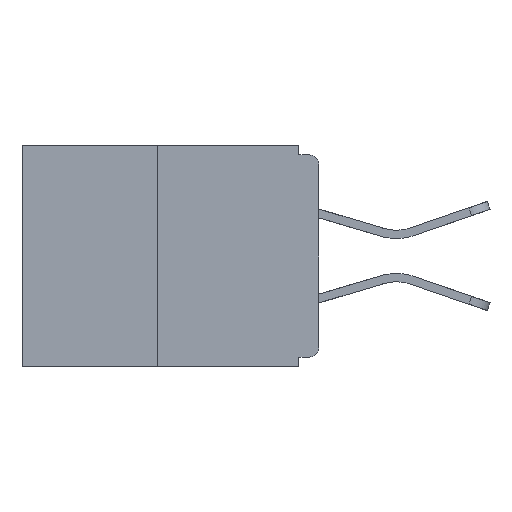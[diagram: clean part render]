
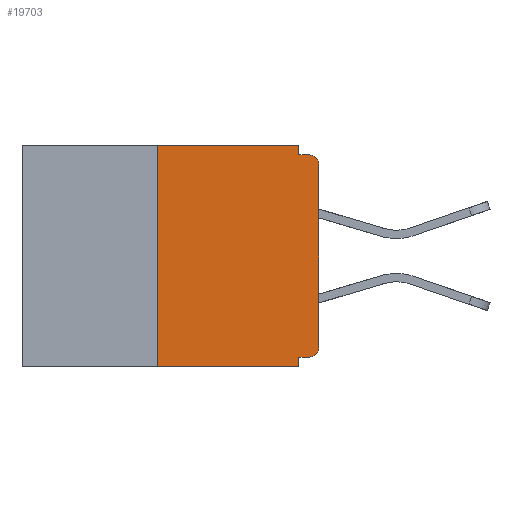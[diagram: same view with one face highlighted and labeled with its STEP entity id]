
A CAD part, left-side view. The second image highlights one B-rep face of the part: STEP entity #19703.
In plain terms, the highlighted planar face has unit normal (-1, 0, 0).
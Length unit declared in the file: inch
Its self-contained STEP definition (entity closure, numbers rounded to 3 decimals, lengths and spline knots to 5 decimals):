
#94 = EDGE_CURVE ( 'NONE', #18329, #1079, #21573, .T. ) ;
#415 = EDGE_LOOP ( 'NONE', ( #25449, #11751, #17042, #2498, #4371, #18953, #9021, #13220, #930, #26460 ) ) ;
#930 = ORIENTED_EDGE ( 'NONE', *, *, #26886, .F. ) ;
#1079 = VERTEX_POINT ( 'NONE', #8988 ) ;
#1086 = DIRECTION ( 'NONE',  ( -1., 0., 0. ) ) ;
#1923 = PLANE ( 'NONE',  #2717 ) ;
#2179 = DIRECTION ( 'NONE',  ( 0., 1., 0. ) ) ;
#2366 = LINE ( 'NONE', #26232, #22673 ) ;
#2498 = ORIENTED_EDGE ( 'NONE', *, *, #21901, .F. ) ;
#2717 = AXIS2_PLACEMENT_3D ( 'NONE', #6183, #8194, #18981 ) ;
#4371 = ORIENTED_EDGE ( 'NONE', *, *, #22115, .F. ) ;
#4397 = CARTESIAN_POINT ( 'NONE',  ( 0., 0.031, 0. ) ) ;
#4636 = CARTESIAN_POINT ( 'NONE',  ( 0., 0.46, -0.343 ) ) ;
#5169 = DIRECTION ( 'NONE',  ( 0., 0., -1. ) ) ;
#5184 = VECTOR ( 'NONE', #20284, 39.37008 ) ;
#5298 = LINE ( 'NONE', #11755, #16798 ) ;
#5553 = DIRECTION ( 'NONE',  ( 0., -1., 0. ) ) ;
#5574 = DIRECTION ( 'NONE',  ( 0., 0., -1. ) ) ;
#6183 = CARTESIAN_POINT ( 'NONE',  ( 0., 0.46, 0. ) ) ;
#6226 = EDGE_CURVE ( 'NONE', #11584, #9669, #20378, .T. ) ;
#6849 = VECTOR ( 'NONE', #2179, 39.37008 ) ;
#7722 = CARTESIAN_POINT ( 'NONE',  ( 0., 0.031, -0.343 ) ) ;
#7896 = AXIS2_PLACEMENT_3D ( 'NONE', #9198, #1086, #5169 ) ;
#8194 = DIRECTION ( 'NONE',  ( 1., 0., 0. ) ) ;
#8895 = EDGE_CURVE ( 'NONE', #9669, #20209, #26828, .T. ) ;
#8988 = CARTESIAN_POINT ( 'NONE',  ( 0., 0.031, -0.015 ) ) ;
#9021 = ORIENTED_EDGE ( 'NONE', *, *, #8895, .T. ) ;
#9198 = CARTESIAN_POINT ( 'NONE',  ( 0., 0.015, -0.03 ) ) ;
#9364 = DIRECTION ( 'NONE',  ( 0., -1., 0. ) ) ;
#9430 = DIRECTION ( 'NONE',  ( 0., 0., 1. ) ) ;
#9669 = VERTEX_POINT ( 'NONE', #10064 ) ;
#9974 = AXIS2_PLACEMENT_3D ( 'NONE', #22675, #10089, #24804 ) ;
#10064 = CARTESIAN_POINT ( 'NONE',  ( 0., 0., -0.313 ) ) ;
#10089 = DIRECTION ( 'NONE',  ( -1., 0., 0. ) ) ;
#10098 = CARTESIAN_POINT ( 'NONE',  ( 0., 0.015, -0.015 ) ) ;
#10408 = VECTOR ( 'NONE', #5574, 39.37008 ) ;
#10593 = DIRECTION ( 'NONE',  ( 0., -1., 0. ) ) ;
#10708 = CARTESIAN_POINT ( 'NONE',  ( 0., 0.015, -0.328 ) ) ;
#11198 = FACE_OUTER_BOUND ( 'NONE', #415, .T. ) ;
#11584 = VERTEX_POINT ( 'NONE', #10708 ) ;
#11751 = ORIENTED_EDGE ( 'NONE', *, *, #12584, .F. ) ;
#11755 = CARTESIAN_POINT ( 'NONE',  ( 0., 0.46, 0. ) ) ;
#12078 = CARTESIAN_POINT ( 'NONE',  ( 0., 0., -0.03 ) ) ;
#12584 = EDGE_CURVE ( 'NONE', #13385, #21059, #2366, .T. ) ;
#13055 = CARTESIAN_POINT ( 'NONE',  ( 0., 0.25, -0.343 ) ) ;
#13220 = ORIENTED_EDGE ( 'NONE', *, *, #23327, .T. ) ;
#13385 = VERTEX_POINT ( 'NONE', #13055 ) ;
#13539 = VERTEX_POINT ( 'NONE', #10098 ) ;
#14301 = CARTESIAN_POINT ( 'NONE',  ( 0., 0., 0. ) ) ;
#16008 = CARTESIAN_POINT ( 'NONE',  ( 0., 0., -0.015 ) ) ;
#16332 = LINE ( 'NONE', #16610, #6849 ) ;
#16610 = CARTESIAN_POINT ( 'NONE',  ( 0., 0., -0.328 ) ) ;
#16798 = VECTOR ( 'NONE', #9364, 39.37008 ) ;
#16844 = VECTOR ( 'NONE', #10593, 39.37008 ) ;
#16888 = VERTEX_POINT ( 'NONE', #23716 ) ;
#17042 = ORIENTED_EDGE ( 'NONE', *, *, #23920, .T. ) ;
#18329 = VERTEX_POINT ( 'NONE', #4397 ) ;
#18516 = DIRECTION ( 'NONE',  ( 0., 0., 1. ) ) ;
#18953 = ORIENTED_EDGE ( 'NONE', *, *, #6226, .T. ) ;
#18981 = DIRECTION ( 'NONE',  ( 0., 0., -1. ) ) ;
#19703 = ADVANCED_FACE ( 'NONE', ( #11198 ), #1923, .F. ) ;
#20209 = VERTEX_POINT ( 'NONE', #12078 ) ;
#20284 = DIRECTION ( 'NONE',  ( 0., 0., -1. ) ) ;
#20378 = CIRCLE ( 'NONE', #9974, 0.015 ) ;
#20770 = CIRCLE ( 'NONE', #7896, 0.015 ) ;
#20812 = CARTESIAN_POINT ( 'NONE',  ( 0., 0.25, 0. ) ) ;
#21059 = VERTEX_POINT ( 'NONE', #20812 ) ;
#21573 = LINE ( 'NONE', #26749, #10408 ) ;
#21901 = EDGE_CURVE ( 'NONE', #26231, #16888, #24234, .T. ) ;
#22115 = EDGE_CURVE ( 'NONE', #11584, #26231, #16332, .T. ) ;
#22438 = LINE ( 'NONE', #4636, #16844 ) ;
#22575 = VECTOR ( 'NONE', #18516, 39.37008 ) ;
#22673 = VECTOR ( 'NONE', #9430, 39.37008 ) ;
#22675 = CARTESIAN_POINT ( 'NONE',  ( 0., 0.015, -0.313 ) ) ;
#23327 = EDGE_CURVE ( 'NONE', #20209, #13539, #20770, .T. ) ;
#23686 = VECTOR ( 'NONE', #5553, 39.37008 ) ;
#23716 = CARTESIAN_POINT ( 'NONE',  ( 0., 0.031, -0.343 ) ) ;
#23920 = EDGE_CURVE ( 'NONE', #13385, #16888, #22438, .T. ) ;
#24234 = LINE ( 'NONE', #7722, #5184 ) ;
#24337 = LINE ( 'NONE', #16008, #23686 ) ;
#24804 = DIRECTION ( 'NONE',  ( 0., 0., -1. ) ) ;
#25449 = ORIENTED_EDGE ( 'NONE', *, *, #25520, .F. ) ;
#25520 = EDGE_CURVE ( 'NONE', #21059, #18329, #5298, .T. ) ;
#26231 = VERTEX_POINT ( 'NONE', #26267 ) ;
#26232 = CARTESIAN_POINT ( 'NONE',  ( 0., 0.25, 0. ) ) ;
#26267 = CARTESIAN_POINT ( 'NONE',  ( 0., 0.031, -0.328 ) ) ;
#26460 = ORIENTED_EDGE ( 'NONE', *, *, #94, .F. ) ;
#26749 = CARTESIAN_POINT ( 'NONE',  ( 0., 0.031, 0. ) ) ;
#26828 = LINE ( 'NONE', #14301, #22575 ) ;
#26886 = EDGE_CURVE ( 'NONE', #1079, #13539, #24337, .T. ) ;
